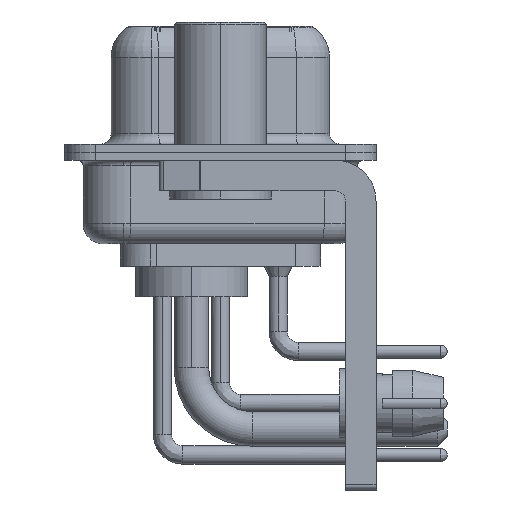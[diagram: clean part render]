
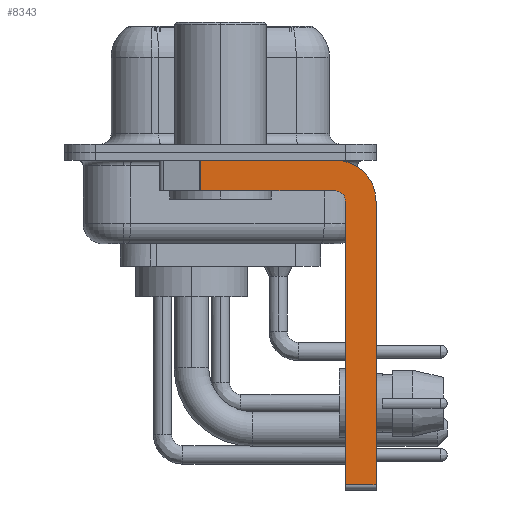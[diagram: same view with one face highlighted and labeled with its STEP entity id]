
A CAD part, left-side view. The second image highlights one B-rep face of the part: STEP entity #8343.
In plain terms, the highlighted planar face has unit normal (-1, 0, 0).
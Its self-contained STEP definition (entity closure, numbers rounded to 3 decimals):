
#772 = AXIS2_PLACEMENT_3D ( 'NONE', #20256, #15228, #26730 ) ;
#844 = CARTESIAN_POINT ( 'NONE',  ( -2.9, 0.978, -1.9 ) ) ;
#1000 = VECTOR ( 'NONE', #36049, 1000. ) ;
#1430 = ORIENTED_EDGE ( 'NONE', *, *, #8999, .F. ) ;
#1494 = VECTOR ( 'NONE', #33285, 1000. ) ;
#1853 = ORIENTED_EDGE ( 'NONE', *, *, #30634, .F. ) ;
#3669 = LINE ( 'NONE', #5905, #29153 ) ;
#4833 = EDGE_CURVE ( 'NONE', #23643, #34716, #22123, .T. ) ;
#4916 = LINE ( 'NONE', #21422, #5590 ) ;
#5471 = EDGE_CURVE ( 'NONE', #22947, #23643, #19637, .T. ) ;
#5590 = VECTOR ( 'NONE', #33107, 1000. ) ;
#5905 = CARTESIAN_POINT ( 'NONE',  ( -2.9, -5.65, -1.9 ) ) ;
#5940 = ORIENTED_EDGE ( 'NONE', *, *, #29602, .T. ) ;
#7172 = VERTEX_POINT ( 'NONE', #13494 ) ;
#8309 = CARTESIAN_POINT ( 'NONE',  ( -2.9, -6.15, -16.6 ) ) ;
#8343 = ADVANCED_FACE ( 'NONE', ( #12253 ), #29297, .F. ) ;
#8871 = DIRECTION ( 'NONE',  ( 0., -1., 0. ) ) ;
#8999 = EDGE_CURVE ( 'NONE', #7172, #17437, #30695, .T. ) ;
#10213 = VERTEX_POINT ( 'NONE', #15248 ) ;
#11078 = EDGE_CURVE ( 'NONE', #22947, #10213, #20732, .T. ) ;
#11151 = AXIS2_PLACEMENT_3D ( 'NONE', #18368, #17987, #29490 ) ;
#12253 = FACE_OUTER_BOUND ( 'NONE', #24434, .T. ) ;
#12858 = VERTEX_POINT ( 'NONE', #844 ) ;
#13494 = CARTESIAN_POINT ( 'NONE',  ( -2.9, 0.978, -0.4 ) ) ;
#14740 = ORIENTED_EDGE ( 'NONE', *, *, #4833, .F. ) ;
#15228 = DIRECTION ( 'NONE',  ( 1., 0., 0. ) ) ;
#15248 = CARTESIAN_POINT ( 'NONE',  ( -2.9, -7.65, -16.35 ) ) ;
#15912 = ORIENTED_EDGE ( 'NONE', *, *, #23953, .F. ) ;
#17123 = CARTESIAN_POINT ( 'NONE',  ( -2.9, -6.15, -16.35 ) ) ;
#17364 = CARTESIAN_POINT ( 'NONE',  ( -2.9, -5.65, -0.4 ) ) ;
#17437 = VERTEX_POINT ( 'NONE', #17364 ) ;
#17987 = DIRECTION ( 'NONE',  ( 1., 0., 0. ) ) ;
#18211 = VECTOR ( 'NONE', #8871, 1000. ) ;
#18368 = CARTESIAN_POINT ( 'NONE',  ( -2.9, -5.65, -2.4 ) ) ;
#18748 = DIRECTION ( 'NONE',  ( -1., 0., 0. ) ) ;
#19202 = VECTOR ( 'NONE', #30934, 1000. ) ;
#19637 = LINE ( 'NONE', #8309, #19202 ) ;
#20196 = DIRECTION ( 'NONE',  ( 0., 1., 0. ) ) ;
#20256 = CARTESIAN_POINT ( 'NONE',  ( -2.9, -5.65, -2.4 ) ) ;
#20732 = LINE ( 'NONE', #32037, #18211 ) ;
#21422 = CARTESIAN_POINT ( 'NONE',  ( -2.9, 0.978, -1.9 ) ) ;
#22041 = CARTESIAN_POINT ( 'NONE',  ( -2.9, -6.15, -2.4 ) ) ;
#22123 = CIRCLE ( 'NONE', #23315, 0.5 ) ;
#22947 = VERTEX_POINT ( 'NONE', #17123 ) ;
#23315 = AXIS2_PLACEMENT_3D ( 'NONE', #23919, #18748, #26890 ) ;
#23643 = VERTEX_POINT ( 'NONE', #22041 ) ;
#23919 = CARTESIAN_POINT ( 'NONE',  ( -2.9, -5.65, -2.4 ) ) ;
#23953 = EDGE_CURVE ( 'NONE', #34716, #12858, #3669, .T. ) ;
#24434 = EDGE_LOOP ( 'NONE', ( #1430, #5940, #15912, #14740, #30501, #29097, #24873, #1853 ) ) ;
#24873 = ORIENTED_EDGE ( 'NONE', *, *, #35471, .F. ) ;
#26730 = DIRECTION ( 'NONE',  ( 0., 0., -1. ) ) ;
#26824 = CIRCLE ( 'NONE', #772, 2. ) ;
#26890 = DIRECTION ( 'NONE',  ( 0., 0., 1. ) ) ;
#28046 = LINE ( 'NONE', #33071, #1000 ) ;
#29097 = ORIENTED_EDGE ( 'NONE', *, *, #11078, .T. ) ;
#29153 = VECTOR ( 'NONE', #20196, 1000. ) ;
#29297 = PLANE ( 'NONE',  #11151 ) ;
#29490 = DIRECTION ( 'NONE',  ( 0., 0., -1. ) ) ;
#29602 = EDGE_CURVE ( 'NONE', #7172, #12858, #4916, .T. ) ;
#30380 = CARTESIAN_POINT ( 'NONE',  ( -2.9, -7.65, -2.4 ) ) ;
#30501 = ORIENTED_EDGE ( 'NONE', *, *, #5471, .F. ) ;
#30634 = EDGE_CURVE ( 'NONE', #17437, #34478, #26824, .T. ) ;
#30695 = LINE ( 'NONE', #35879, #1494 ) ;
#30934 = DIRECTION ( 'NONE',  ( 0., 0., 1. ) ) ;
#32037 = CARTESIAN_POINT ( 'NONE',  ( -2.9, -5.65, -16.35 ) ) ;
#33071 = CARTESIAN_POINT ( 'NONE',  ( -2.9, -7.65, -2.4 ) ) ;
#33107 = DIRECTION ( 'NONE',  ( 0., 0., -1. ) ) ;
#33285 = DIRECTION ( 'NONE',  ( 0., -1., 0. ) ) ;
#34478 = VERTEX_POINT ( 'NONE', #30380 ) ;
#34716 = VERTEX_POINT ( 'NONE', #34994 ) ;
#34994 = CARTESIAN_POINT ( 'NONE',  ( -2.9, -5.65, -1.9 ) ) ;
#35471 = EDGE_CURVE ( 'NONE', #34478, #10213, #28046, .T. ) ;
#35879 = CARTESIAN_POINT ( 'NONE',  ( -2.9, 3., -0.4 ) ) ;
#36049 = DIRECTION ( 'NONE',  ( 0., 0., -1. ) ) ;
